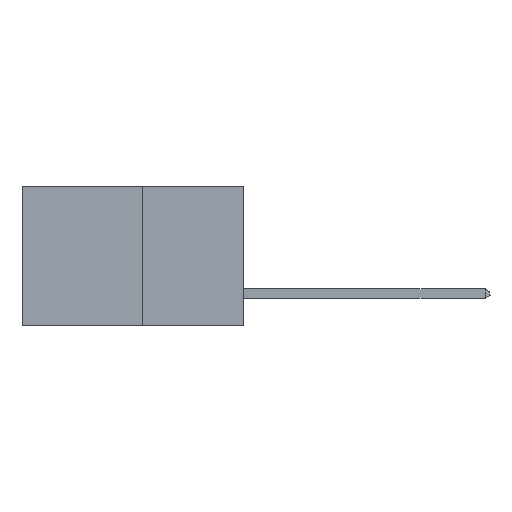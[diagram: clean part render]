
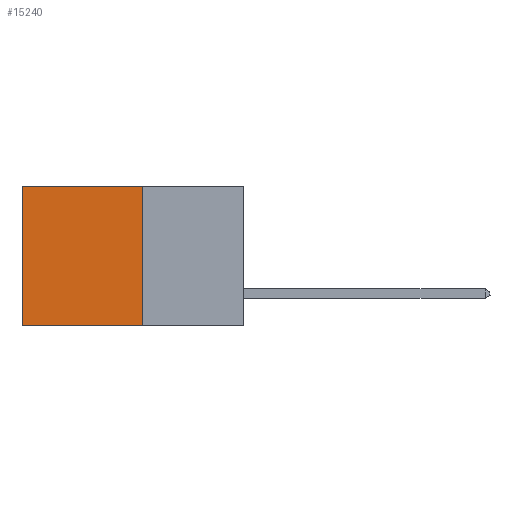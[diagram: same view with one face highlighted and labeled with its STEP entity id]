
A CAD part, left-side view. The second image highlights one B-rep face of the part: STEP entity #15240.
In plain terms, the highlighted planar face has unit normal (-1, 0, 0).
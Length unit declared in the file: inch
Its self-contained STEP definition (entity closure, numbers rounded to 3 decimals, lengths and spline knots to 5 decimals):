
#2328 = LINE ( 'NONE', #18043, #14338 ) ;
#2809 = VERTEX_POINT ( 'NONE', #11940 ) ;
#3133 = EDGE_CURVE ( 'NONE', #3938, #23429, #28807, .T. ) ;
#3761 = FACE_OUTER_BOUND ( 'NONE', #11534, .T. ) ;
#3938 = VERTEX_POINT ( 'NONE', #11002 ) ;
#4516 = EDGE_CURVE ( 'NONE', #2809, #23429, #2328, .T. ) ;
#4653 = PLANE ( 'NONE',  #15516 ) ;
#5243 = LINE ( 'NONE', #9580, #17918 ) ;
#5659 = ORIENTED_EDGE ( 'NONE', *, *, #27204, .F. ) ;
#5665 = VERTEX_POINT ( 'NONE', #23514 ) ;
#9421 = CARTESIAN_POINT ( 'NONE',  ( 0.277, 0.27, -0.37 ) ) ;
#9580 = CARTESIAN_POINT ( 'NONE',  ( 0.277, 0.27, 0. ) ) ;
#9862 = VECTOR ( 'NONE', #27376, 39.37008 ) ;
#11002 = CARTESIAN_POINT ( 'NONE',  ( 0.277, 0.27, -0.37 ) ) ;
#11534 = EDGE_LOOP ( 'NONE', ( #24567, #29379, #5659, #25821 ) ) ;
#11835 = DIRECTION ( 'NONE',  ( 0., 0., -1. ) ) ;
#11940 = CARTESIAN_POINT ( 'NONE',  ( 0.277, 0.59, 0. ) ) ;
#14338 = VECTOR ( 'NONE', #17617, 39.37008 ) ;
#14395 = DIRECTION ( 'NONE',  ( 0., 1., 0. ) ) ;
#15240 = ADVANCED_FACE ( 'NONE', ( #3761 ), #4653, .F. ) ;
#15516 = AXIS2_PLACEMENT_3D ( 'NONE', #9421, #26071, #11835 ) ;
#16379 = CARTESIAN_POINT ( 'NONE',  ( 0.277, 0.59, -0.37 ) ) ;
#17617 = DIRECTION ( 'NONE',  ( 0., 0., -1. ) ) ;
#17918 = VECTOR ( 'NONE', #14395, 39.37008 ) ;
#18043 = CARTESIAN_POINT ( 'NONE',  ( 0.277, 0.59, -0.37 ) ) ;
#19251 = DIRECTION ( 'NONE',  ( 0., 0., -1. ) ) ;
#20822 = EDGE_CURVE ( 'NONE', #5665, #2809, #5243, .T. ) ;
#20880 = VECTOR ( 'NONE', #19251, 39.37008 ) ;
#21620 = LINE ( 'NONE', #28620, #20880 ) ;
#23429 = VERTEX_POINT ( 'NONE', #16379 ) ;
#23514 = CARTESIAN_POINT ( 'NONE',  ( 0.277, 0.27, 0. ) ) ;
#24567 = ORIENTED_EDGE ( 'NONE', *, *, #4516, .T. ) ;
#25821 = ORIENTED_EDGE ( 'NONE', *, *, #20822, .T. ) ;
#26071 = DIRECTION ( 'NONE',  ( 1., 0., 0. ) ) ;
#27204 = EDGE_CURVE ( 'NONE', #5665, #3938, #21620, .T. ) ;
#27376 = DIRECTION ( 'NONE',  ( 0., 1., 0. ) ) ;
#28620 = CARTESIAN_POINT ( 'NONE',  ( 0.277, 0.27, -0.37 ) ) ;
#28807 = LINE ( 'NONE', #29295, #9862 ) ;
#29295 = CARTESIAN_POINT ( 'NONE',  ( 0.277, 0.27, -0.37 ) ) ;
#29379 = ORIENTED_EDGE ( 'NONE', *, *, #3133, .F. ) ;
